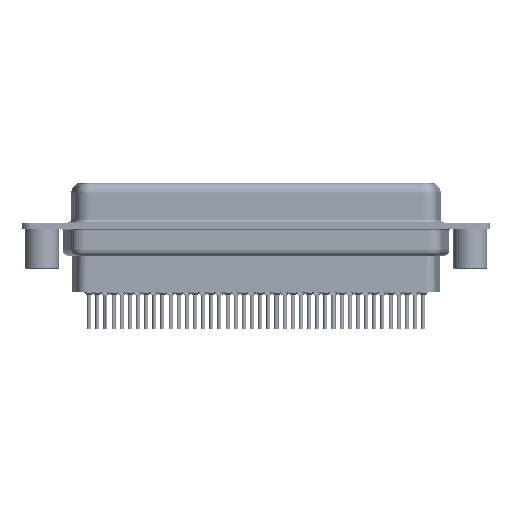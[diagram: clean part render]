
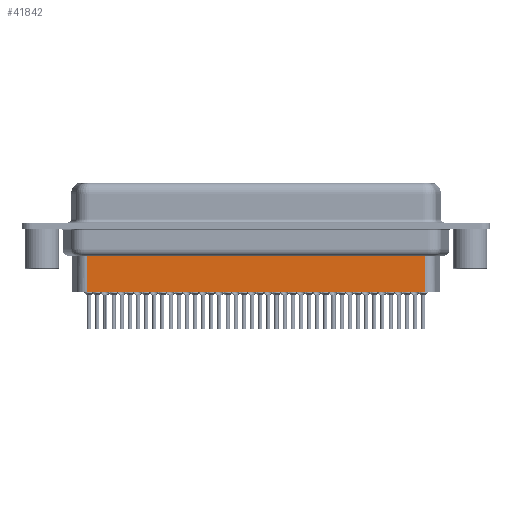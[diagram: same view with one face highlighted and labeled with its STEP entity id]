
A CAD part, front view. The second image highlights one B-rep face of the part: STEP entity #41842.
In plain terms, the highlighted planar face has unit normal (0, -1, 0).
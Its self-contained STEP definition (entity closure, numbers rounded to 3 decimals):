
#294 = VERTEX_POINT ( 'NONE', #14942 ) ;
#1202 = DIRECTION ( 'NONE',  ( 0., 0., -1. ) ) ;
#2360 = ORIENTED_EDGE ( 'NONE', *, *, #43251, .T. ) ;
#3043 = PLANE ( 'NONE',  #24746 ) ;
#3665 = LINE ( 'NONE', #43581, #26039 ) ;
#4856 = CARTESIAN_POINT ( 'NONE',  ( 6.706, -3.5, -9.85 ) ) ;
#7064 = VECTOR ( 'NONE', #30606, 1000. ) ;
#8974 = LINE ( 'NONE', #23616, #7064 ) ;
#9392 = DIRECTION ( 'NONE',  ( 1., 0., 0. ) ) ;
#10922 = VERTEX_POINT ( 'NONE', #38806 ) ;
#10975 = EDGE_CURVE ( 'NONE', #40329, #10922, #3665, .T. ) ;
#12722 = DIRECTION ( 'NONE',  ( -1., 0., 0. ) ) ;
#14532 = LINE ( 'NONE', #26087, #44823 ) ;
#14942 = CARTESIAN_POINT ( 'NONE',  ( 6.706, -3.5, -4.097 ) ) ;
#16576 = FACE_OUTER_BOUND ( 'NONE', #44554, .T. ) ;
#20501 = EDGE_CURVE ( 'NONE', #40329, #294, #31006, .T. ) ;
#23616 = CARTESIAN_POINT ( 'NONE',  ( 6.706, -3.5, -9.85 ) ) ;
#24746 = AXIS2_PLACEMENT_3D ( 'NONE', #45456, #27661, #9392 ) ;
#26039 = VECTOR ( 'NONE', #1202, 1000. ) ;
#26087 = CARTESIAN_POINT ( 'NONE',  ( 6.706, -3.5, -3.1 ) ) ;
#27661 = DIRECTION ( 'NONE',  ( 0., -1., 0. ) ) ;
#29722 = ORIENTED_EDGE ( 'NONE', *, *, #41445, .F. ) ;
#30324 = ORIENTED_EDGE ( 'NONE', *, *, #20501, .T. ) ;
#30606 = DIRECTION ( 'NONE',  ( -1., 0., 0. ) ) ;
#31006 = LINE ( 'NONE', #45661, #34324 ) ;
#33970 = VERTEX_POINT ( 'NONE', #4856 ) ;
#34324 = VECTOR ( 'NONE', #12722, 1000. ) ;
#36320 = ORIENTED_EDGE ( 'NONE', *, *, #10975, .F. ) ;
#37153 = DIRECTION ( 'NONE',  ( 0., 0., -1. ) ) ;
#38806 = CARTESIAN_POINT ( 'NONE',  ( 56.794, -3.5, -9.85 ) ) ;
#40329 = VERTEX_POINT ( 'NONE', #43810 ) ;
#41445 = EDGE_CURVE ( 'NONE', #10922, #33970, #8974, .T. ) ;
#41842 = ADVANCED_FACE ( 'NONE', ( #16576 ), #3043, .T. ) ;
#43251 = EDGE_CURVE ( 'NONE', #294, #33970, #14532, .T. ) ;
#43581 = CARTESIAN_POINT ( 'NONE',  ( 56.794, -3.5, -3.1 ) ) ;
#43810 = CARTESIAN_POINT ( 'NONE',  ( 56.794, -3.5, -4.097 ) ) ;
#44554 = EDGE_LOOP ( 'NONE', ( #36320, #30324, #2360, #29722 ) ) ;
#44823 = VECTOR ( 'NONE', #37153, 1000. ) ;
#45456 = CARTESIAN_POINT ( 'NONE',  ( 6.706, -3.5, -3.1 ) ) ;
#45661 = CARTESIAN_POINT ( 'NONE',  ( 6.459, -3.5, -4.097 ) ) ;
